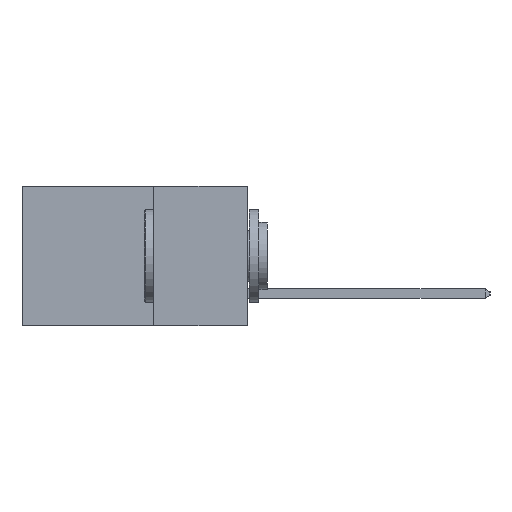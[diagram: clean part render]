
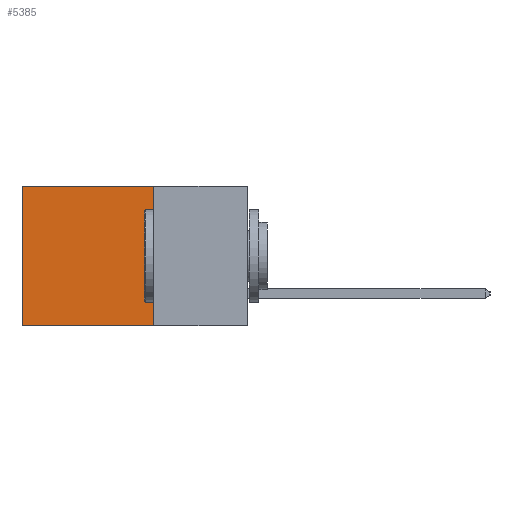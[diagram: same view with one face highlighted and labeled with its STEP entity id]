
A CAD part, left-side view. The second image highlights one B-rep face of the part: STEP entity #5385.
In plain terms, the highlighted planar face has unit normal (-1, 0, 0).
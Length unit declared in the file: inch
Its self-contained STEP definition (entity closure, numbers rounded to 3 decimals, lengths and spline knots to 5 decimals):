
#635 = LINE ( 'NONE', #10754, #9491 ) ;
#1825 = EDGE_CURVE ( 'NONE', #14937, #6273, #2896, .T. ) ;
#2151 = CARTESIAN_POINT ( 'NONE',  ( 0.2615, 0.6, 0. ) ) ;
#2526 = VECTOR ( 'NONE', #6879, 39.37008 ) ;
#2557 = CARTESIAN_POINT ( 'NONE',  ( 0.2615, 0.25, 0. ) ) ;
#2896 = LINE ( 'NONE', #7620, #2526 ) ;
#3366 = DIRECTION ( 'NONE',  ( 0., 1., 0. ) ) ;
#4850 = ORIENTED_EDGE ( 'NONE', *, *, #8423, .F. ) ;
#5375 = VECTOR ( 'NONE', #3366, 39.37008 ) ;
#5385 = ADVANCED_FACE ( 'NONE', ( #8314 ), #7981, .F. ) ;
#5962 = LINE ( 'NONE', #13885, #14858 ) ;
#6273 = VERTEX_POINT ( 'NONE', #2151 ) ;
#6312 = ORIENTED_EDGE ( 'NONE', *, *, #8543, .F. ) ;
#6511 = ORIENTED_EDGE ( 'NONE', *, *, #1825, .T. ) ;
#6879 = DIRECTION ( 'NONE',  ( 0., 1., 0. ) ) ;
#6946 = DIRECTION ( 'NONE',  ( 0., 0., -1. ) ) ;
#6981 = VERTEX_POINT ( 'NONE', #11522 ) ;
#7620 = CARTESIAN_POINT ( 'NONE',  ( 0.2615, 0.25, 0. ) ) ;
#7716 = EDGE_CURVE ( 'NONE', #6273, #6981, #5962, .T. ) ;
#7821 = DIRECTION ( 'NONE',  ( 0., 0., -1. ) ) ;
#7854 = DIRECTION ( 'NONE',  ( 1., 0., 0. ) ) ;
#7966 = CARTESIAN_POINT ( 'NONE',  ( 0.2615, 0.25, -0.37 ) ) ;
#7981 = PLANE ( 'NONE',  #9636 ) ;
#8314 = FACE_OUTER_BOUND ( 'NONE', #11796, .T. ) ;
#8423 = EDGE_CURVE ( 'NONE', #13661, #6981, #14336, .T. ) ;
#8543 = EDGE_CURVE ( 'NONE', #14937, #13661, #635, .T. ) ;
#9491 = VECTOR ( 'NONE', #15248, 39.37008 ) ;
#9636 = AXIS2_PLACEMENT_3D ( 'NONE', #7966, #7854, #7821 ) ;
#10754 = CARTESIAN_POINT ( 'NONE',  ( 0.2615, 0.25, -0.37 ) ) ;
#11522 = CARTESIAN_POINT ( 'NONE',  ( 0.2615, 0.6, -0.37 ) ) ;
#11796 = EDGE_LOOP ( 'NONE', ( #14286, #4850, #6312, #6511 ) ) ;
#13661 = VERTEX_POINT ( 'NONE', #14084 ) ;
#13885 = CARTESIAN_POINT ( 'NONE',  ( 0.2615, 0.6, -0.37 ) ) ;
#14084 = CARTESIAN_POINT ( 'NONE',  ( 0.2615, 0.25, -0.37 ) ) ;
#14286 = ORIENTED_EDGE ( 'NONE', *, *, #7716, .T. ) ;
#14336 = LINE ( 'NONE', #15050, #5375 ) ;
#14858 = VECTOR ( 'NONE', #6946, 39.37008 ) ;
#14937 = VERTEX_POINT ( 'NONE', #2557 ) ;
#15050 = CARTESIAN_POINT ( 'NONE',  ( 0.2615, 0.25, -0.37 ) ) ;
#15248 = DIRECTION ( 'NONE',  ( 0., 0., -1. ) ) ;
